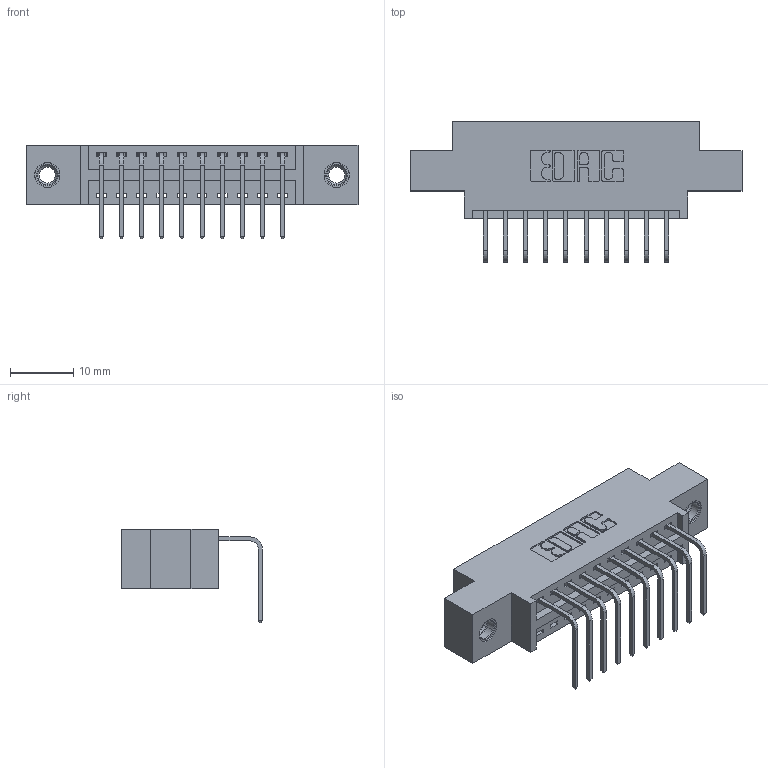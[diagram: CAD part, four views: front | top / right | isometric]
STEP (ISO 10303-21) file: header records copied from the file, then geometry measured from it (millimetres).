
FILE_DESCRIPTION (( 'STEP AP203' ), '1' );
FILE_NAME ('396-010-558-607.STEP', '2019-11-01T05:27:54', ( '' ), ( '' ), 'SwSTEP 2.0', 'SolidWorks 2016', '' );
FILE_SCHEMA (( 'CONFIG_CONTROL_DESIGN' ));
Length unit declared in the file: inch
Products named in the file (4): 346 Part_0.170 Offset - 0.156 Dia-TI; 345-292-001_558 Tail - 2; 345-250-001_345-250-005-103; 396-010-558-607
Assembly tree (13 placements, depth 2):
  396-010-558-607
    346 Part_0.170 Offset - 0.156 Dia-TI
    345-292-001_558 Tail - 2  x10
    345-250-001_345-250-005-103  x2
Bounding box: 52.32 x 22.16 x 14.73 mm (x, y, z)
Volume: 4653.3 mm3; surface area: 5864.4 mm2
Topology: 13 solids, 13 shells, 786 faces, 2297 edges, 1510 vertices
Faces by surface type: plane 532, cylinder 238, cone 12, torus 4
Entity records: 11916 total; most frequent: CARTESIAN_POINT 2037, ORIENTED_EDGE 1974, DIRECTION 1861, EDGE_CURVE 987, VECTOR 795, LINE 795, VERTEX_POINT 652, AXIS2_PLACEMENT_3D 533
